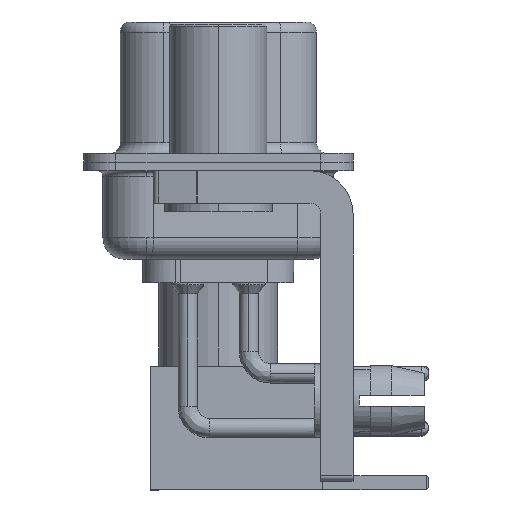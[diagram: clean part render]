
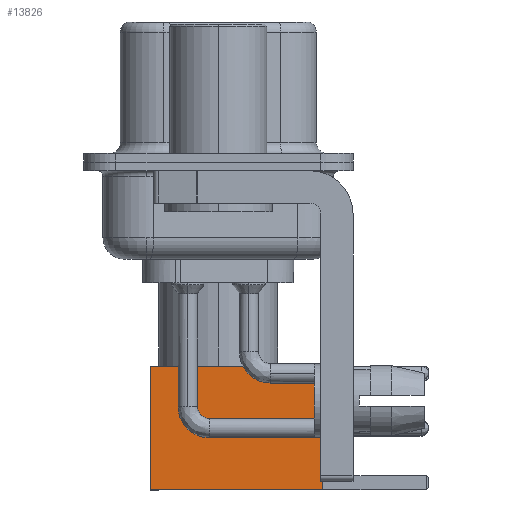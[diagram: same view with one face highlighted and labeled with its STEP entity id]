
A CAD part, left-side view. The second image highlights one B-rep face of the part: STEP entity #13826.
In plain terms, the highlighted face is planar.
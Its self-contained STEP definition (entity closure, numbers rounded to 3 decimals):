
#628 = DIRECTION ( 'NONE',  ( 0., 0., -1. ) ) ;
#1209 = CARTESIAN_POINT ( 'NONE',  ( 0., 2.875, 0. ) ) ;
#2341 = CARTESIAN_POINT ( 'NONE',  ( 2.875, 2.875, 8. ) ) ;
#4056 = LINE ( 'NONE', #14739, #23048 ) ;
#4552 = VECTOR ( 'NONE', #628, 1000. ) ;
#4674 = PLANE ( 'NONE',  #27418 ) ;
#6406 = CARTESIAN_POINT ( 'NONE',  ( 2.875, 2.875, 0. ) ) ;
#6867 = LINE ( 'NONE', #21987, #4552 ) ;
#7392 = CARTESIAN_POINT ( 'NONE',  ( -2.875, 2.875, 8. ) ) ;
#8772 = EDGE_CURVE ( 'NONE', #15438, #18725, #6867, .T. ) ;
#8979 = DIRECTION ( 'NONE',  ( 0., 0., 1. ) ) ;
#9036 = ORIENTED_EDGE ( 'NONE', *, *, #19179, .T. ) ;
#9410 = LINE ( 'NONE', #1209, #17353 ) ;
#10554 = EDGE_LOOP ( 'NONE', ( #18652, #9036, #21073, #23336 ) ) ;
#10898 = VECTOR ( 'NONE', #22899, 1000. ) ;
#13139 = CARTESIAN_POINT ( 'NONE',  ( 2.875, 2.875, 0. ) ) ;
#13826 = ADVANCED_FACE ( 'NONE', ( #15355 ), #4674, .T. ) ;
#14739 = CARTESIAN_POINT ( 'NONE',  ( 0., 2.875, 8. ) ) ;
#15355 = FACE_OUTER_BOUND ( 'NONE', #10554, .T. ) ;
#15438 = VERTEX_POINT ( 'NONE', #7392 ) ;
#15991 = VERTEX_POINT ( 'NONE', #26491 ) ;
#16962 = DIRECTION ( 'NONE',  ( -1., 0., 0. ) ) ;
#17353 = VECTOR ( 'NONE', #20366, 1000. ) ;
#17892 = CARTESIAN_POINT ( 'NONE',  ( -2.875, 2.875, 0. ) ) ;
#18652 = ORIENTED_EDGE ( 'NONE', *, *, #22059, .T. ) ;
#18725 = VERTEX_POINT ( 'NONE', #17892 ) ;
#18752 = LINE ( 'NONE', #6406, #10898 ) ;
#19179 = EDGE_CURVE ( 'NONE', #15991, #18725, #9410, .T. ) ;
#20366 = DIRECTION ( 'NONE',  ( -1., 0., 0. ) ) ;
#21073 = ORIENTED_EDGE ( 'NONE', *, *, #8772, .F. ) ;
#21605 = DIRECTION ( 'NONE',  ( 0., 1., 0. ) ) ;
#21987 = CARTESIAN_POINT ( 'NONE',  ( -2.875, 2.875, 0. ) ) ;
#22059 = EDGE_CURVE ( 'NONE', #22912, #15991, #18752, .T. ) ;
#22899 = DIRECTION ( 'NONE',  ( 0., 0., -1. ) ) ;
#22912 = VERTEX_POINT ( 'NONE', #2341 ) ;
#23048 = VECTOR ( 'NONE', #16962, 1000. ) ;
#23336 = ORIENTED_EDGE ( 'NONE', *, *, #26616, .F. ) ;
#26491 = CARTESIAN_POINT ( 'NONE',  ( 2.875, 2.875, 0. ) ) ;
#26616 = EDGE_CURVE ( 'NONE', #22912, #15438, #4056, .T. ) ;
#27418 = AXIS2_PLACEMENT_3D ( 'NONE', #13139, #21605, #8979 ) ;
